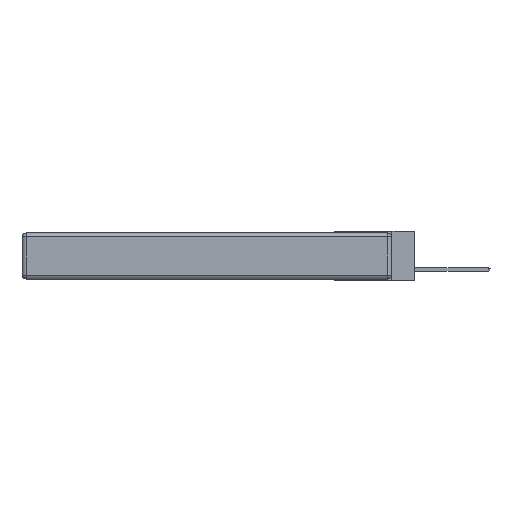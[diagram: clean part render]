
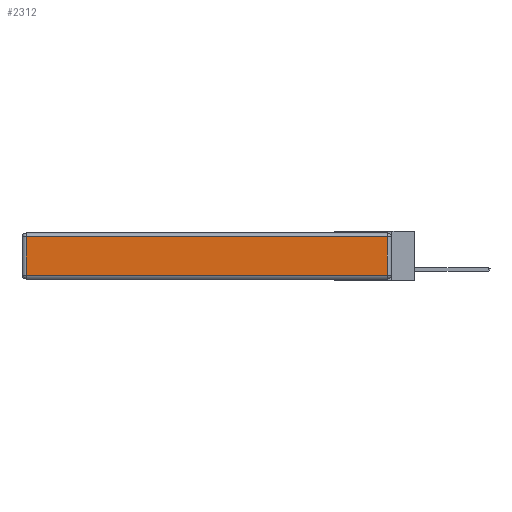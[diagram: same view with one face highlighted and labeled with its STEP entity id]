
A CAD part, left-side view. The second image highlights one B-rep face of the part: STEP entity #2312.
In plain terms, the highlighted planar face has unit normal (-1, 0, 0).
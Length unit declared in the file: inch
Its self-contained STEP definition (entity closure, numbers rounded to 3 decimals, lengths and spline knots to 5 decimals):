
#525 = DIRECTION ( 'NONE',  ( 0., 0., 1. ) ) ;
#786 = CARTESIAN_POINT ( 'NONE',  ( 0., 0., -0.343 ) ) ;
#1003 = DIRECTION ( 'NONE',  ( 0., 0., 1. ) ) ;
#1924 = ORIENTED_EDGE ( 'NONE', *, *, #25962, .T. ) ;
#1968 = VECTOR ( 'NONE', #3983, 39.37008 ) ;
#2312 = ADVANCED_FACE ( 'NONE', ( #23961 ), #25209, .T. ) ;
#3983 = DIRECTION ( 'NONE',  ( 0., -1., 0. ) ) ;
#4468 = EDGE_CURVE ( 'NONE', #13813, #5050, #6057, .T. ) ;
#4515 = VECTOR ( 'NONE', #1003, 39.37008 ) ;
#4543 = AXIS2_PLACEMENT_3D ( 'NONE', #786, #15212, #525 ) ;
#5050 = VERTEX_POINT ( 'NONE', #20640 ) ;
#5561 = LINE ( 'NONE', #16698, #13692 ) ;
#6057 = LINE ( 'NONE', #8695, #21914 ) ;
#6339 = DIRECTION ( 'NONE',  ( 0., 0., -1. ) ) ;
#7184 = CARTESIAN_POINT ( 'NONE',  ( 0., 0.03, -0.313 ) ) ;
#8585 = CARTESIAN_POINT ( 'NONE',  ( 0., 2.72, -0.313 ) ) ;
#8695 = CARTESIAN_POINT ( 'NONE',  ( 0., 2.75, -0.03 ) ) ;
#8742 = ORIENTED_EDGE ( 'NONE', *, *, #17548, .T. ) ;
#11661 = CARTESIAN_POINT ( 'NONE',  ( 0., 0.03, -0.343 ) ) ;
#11751 = ORIENTED_EDGE ( 'NONE', *, *, #4468, .T. ) ;
#13692 = VECTOR ( 'NONE', #6339, 39.37008 ) ;
#13813 = VERTEX_POINT ( 'NONE', #26235 ) ;
#14394 = CARTESIAN_POINT ( 'NONE',  ( 0., 0., -0.313 ) ) ;
#15212 = DIRECTION ( 'NONE',  ( -1., 0., 0. ) ) ;
#15551 = LINE ( 'NONE', #14394, #1968 ) ;
#16698 = CARTESIAN_POINT ( 'NONE',  ( 0., 2.72, -0.343 ) ) ;
#17548 = EDGE_CURVE ( 'NONE', #21545, #19871, #15551, .T. ) ;
#19871 = VERTEX_POINT ( 'NONE', #7184 ) ;
#20543 = ORIENTED_EDGE ( 'NONE', *, *, #25631, .T. ) ;
#20640 = CARTESIAN_POINT ( 'NONE',  ( 0., 2.72, -0.03 ) ) ;
#21545 = VERTEX_POINT ( 'NONE', #8585 ) ;
#21914 = VECTOR ( 'NONE', #23109, 39.37008 ) ;
#22030 = LINE ( 'NONE', #11661, #4515 ) ;
#23109 = DIRECTION ( 'NONE',  ( 0., 1., 0. ) ) ;
#23961 = FACE_OUTER_BOUND ( 'NONE', #25786, .T. ) ;
#25209 = PLANE ( 'NONE',  #4543 ) ;
#25631 = EDGE_CURVE ( 'NONE', #5050, #21545, #5561, .T. ) ;
#25786 = EDGE_LOOP ( 'NONE', ( #8742, #1924, #11751, #20543 ) ) ;
#25962 = EDGE_CURVE ( 'NONE', #19871, #13813, #22030, .T. ) ;
#26235 = CARTESIAN_POINT ( 'NONE',  ( 0., 0.03, -0.03 ) ) ;
